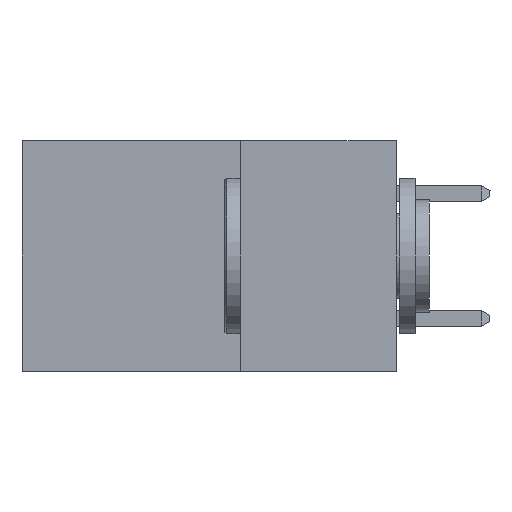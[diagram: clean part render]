
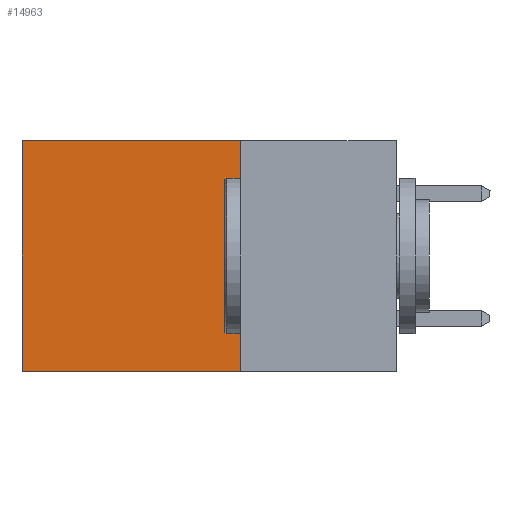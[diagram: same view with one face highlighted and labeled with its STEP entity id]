
A CAD part, left-side view. The second image highlights one B-rep face of the part: STEP entity #14963.
In plain terms, the highlighted planar face has unit normal (-1, 0, 0).
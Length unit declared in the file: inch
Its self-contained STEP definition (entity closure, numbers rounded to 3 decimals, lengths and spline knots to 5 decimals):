
#28 = VERTEX_POINT ( 'NONE', #22363 ) ;
#224 = LINE ( 'NONE', #9862, #23393 ) ;
#292 = DIRECTION ( 'NONE',  ( 1., 0., 0. ) ) ;
#1118 = VECTOR ( 'NONE', #14330, 39.37008 ) ;
#2675 = ORIENTED_EDGE ( 'NONE', *, *, #13869, .F. ) ;
#2960 = FACE_OUTER_BOUND ( 'NONE', #17398, .T. ) ;
#3102 = ORIENTED_EDGE ( 'NONE', *, *, #3264, .F. ) ;
#3264 = EDGE_CURVE ( 'NONE', #14893, #27695, #4070, .T. ) ;
#4070 = LINE ( 'NONE', #15693, #8554 ) ;
#4627 = PLANE ( 'NONE',  #15556 ) ;
#4642 = VERTEX_POINT ( 'NONE', #25305 ) ;
#6496 = ORIENTED_EDGE ( 'NONE', *, *, #26656, .T. ) ;
#6655 = CARTESIAN_POINT ( 'NONE',  ( 0.298, 0.25, -0.37 ) ) ;
#7857 = VECTOR ( 'NONE', #15820, 39.37008 ) ;
#8554 = VECTOR ( 'NONE', #15508, 39.37008 ) ;
#9862 = CARTESIAN_POINT ( 'NONE',  ( 0.298, 0.6, 0. ) ) ;
#12175 = CARTESIAN_POINT ( 'NONE',  ( 0.298, 0.25, 0. ) ) ;
#12785 = LINE ( 'NONE', #12175, #1118 ) ;
#13417 = CARTESIAN_POINT ( 'NONE',  ( 0.298, 0.25, 0. ) ) ;
#13653 = LINE ( 'NONE', #24393, #7857 ) ;
#13869 = EDGE_CURVE ( 'NONE', #28, #14893, #13653, .T. ) ;
#14330 = DIRECTION ( 'NONE',  ( 0., 1., 0. ) ) ;
#14893 = VERTEX_POINT ( 'NONE', #6655 ) ;
#14963 = ADVANCED_FACE ( 'NONE', ( #2960 ), #4627, .F. ) ;
#15508 = DIRECTION ( 'NONE',  ( 0., 1., 0. ) ) ;
#15556 = AXIS2_PLACEMENT_3D ( 'NONE', #13417, #292, #15614 ) ;
#15614 = DIRECTION ( 'NONE',  ( 0., 0., -1. ) ) ;
#15693 = CARTESIAN_POINT ( 'NONE',  ( 0.298, 0.25, -0.37 ) ) ;
#15820 = DIRECTION ( 'NONE',  ( 0., 0., -1. ) ) ;
#17398 = EDGE_LOOP ( 'NONE', ( #6496, #3102, #2675, #19883 ) ) ;
#19883 = ORIENTED_EDGE ( 'NONE', *, *, #20813, .T. ) ;
#20813 = EDGE_CURVE ( 'NONE', #28, #4642, #12785, .T. ) ;
#22363 = CARTESIAN_POINT ( 'NONE',  ( 0.298, 0.25, 0. ) ) ;
#23265 = CARTESIAN_POINT ( 'NONE',  ( 0.298, 0.6, -0.37 ) ) ;
#23393 = VECTOR ( 'NONE', #24969, 39.37008 ) ;
#24393 = CARTESIAN_POINT ( 'NONE',  ( 0.298, 0.25, 0. ) ) ;
#24969 = DIRECTION ( 'NONE',  ( 0., 0., -1. ) ) ;
#25305 = CARTESIAN_POINT ( 'NONE',  ( 0.298, 0.6, 0. ) ) ;
#26656 = EDGE_CURVE ( 'NONE', #4642, #27695, #224, .T. ) ;
#27695 = VERTEX_POINT ( 'NONE', #23265 ) ;
